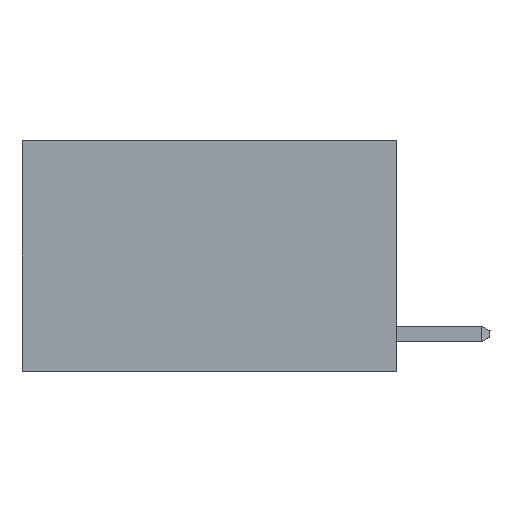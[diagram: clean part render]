
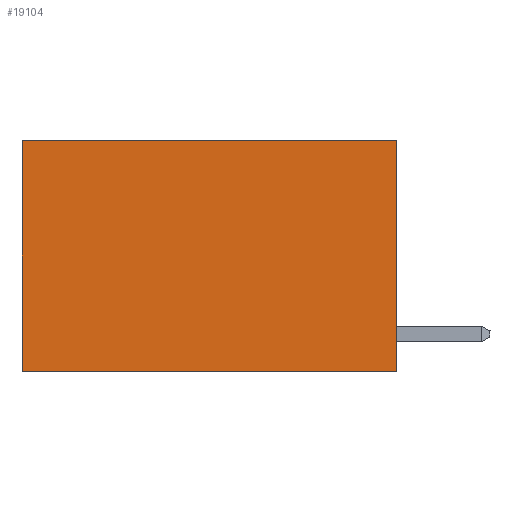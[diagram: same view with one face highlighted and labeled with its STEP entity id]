
A CAD part, left-side view. The second image highlights one B-rep face of the part: STEP entity #19104.
In plain terms, the highlighted planar face has unit normal (-1, 0, 0).
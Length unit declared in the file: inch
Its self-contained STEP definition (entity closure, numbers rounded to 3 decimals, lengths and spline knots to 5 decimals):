
#360 = VERTEX_POINT ( 'NONE', #3849 ) ;
#455 = VERTEX_POINT ( 'NONE', #20634 ) ;
#544 = VECTOR ( 'NONE', #22483, 39.37008 ) ;
#897 = DIRECTION ( 'NONE',  ( 0., 1., 0. ) ) ;
#1497 = ORIENTED_EDGE ( 'NONE', *, *, #5236, .T. ) ;
#1643 = ORIENTED_EDGE ( 'NONE', *, *, #20049, .F. ) ;
#1742 = DIRECTION ( 'NONE',  ( 0., 0., -1. ) ) ;
#2831 = DIRECTION ( 'NONE',  ( 0., 0., -1. ) ) ;
#3849 = CARTESIAN_POINT ( 'NONE',  ( 0.2625, 0., -0.37 ) ) ;
#4881 = ORIENTED_EDGE ( 'NONE', *, *, #5861, .T. ) ;
#5236 = EDGE_CURVE ( 'NONE', #24550, #455, #22586, .T. ) ;
#5306 = FACE_OUTER_BOUND ( 'NONE', #16448, .T. ) ;
#5861 = EDGE_CURVE ( 'NONE', #455, #8704, #11756, .T. ) ;
#6085 = VECTOR ( 'NONE', #17702, 39.37008 ) ;
#8704 = VERTEX_POINT ( 'NONE', #14972 ) ;
#11299 = PLANE ( 'NONE',  #25858 ) ;
#11756 = LINE ( 'NONE', #19719, #6085 ) ;
#13417 = CARTESIAN_POINT ( 'NONE',  ( 0.2625, 0., 0. ) ) ;
#13444 = EDGE_CURVE ( 'NONE', #360, #8704, #17443, .T. ) ;
#13879 = LINE ( 'NONE', #26933, #24299 ) ;
#14972 = CARTESIAN_POINT ( 'NONE',  ( 0.2625, 0.6, -0.37 ) ) ;
#15527 = DIRECTION ( 'NONE',  ( 1., 0., 0. ) ) ;
#16113 = CARTESIAN_POINT ( 'NONE',  ( 0.2625, 0., -0.37 ) ) ;
#16448 = EDGE_LOOP ( 'NONE', ( #4881, #17006, #1643, #1497 ) ) ;
#17006 = ORIENTED_EDGE ( 'NONE', *, *, #13444, .F. ) ;
#17443 = LINE ( 'NONE', #16113, #544 ) ;
#17694 = CARTESIAN_POINT ( 'NONE',  ( 0.2625, 0., 0. ) ) ;
#17702 = DIRECTION ( 'NONE',  ( 0., 0., -1. ) ) ;
#19104 = ADVANCED_FACE ( 'NONE', ( #5306 ), #11299, .F. ) ;
#19719 = CARTESIAN_POINT ( 'NONE',  ( 0.2625, 0.6, 0. ) ) ;
#19832 = CARTESIAN_POINT ( 'NONE',  ( 0.2625, 0., 0. ) ) ;
#20049 = EDGE_CURVE ( 'NONE', #24550, #360, #13879, .T. ) ;
#20634 = CARTESIAN_POINT ( 'NONE',  ( 0.2625, 0.6, 0. ) ) ;
#21947 = VECTOR ( 'NONE', #897, 39.37008 ) ;
#22483 = DIRECTION ( 'NONE',  ( 0., 1., 0. ) ) ;
#22586 = LINE ( 'NONE', #19832, #21947 ) ;
#24299 = VECTOR ( 'NONE', #1742, 39.37008 ) ;
#24550 = VERTEX_POINT ( 'NONE', #17694 ) ;
#25858 = AXIS2_PLACEMENT_3D ( 'NONE', #13417, #15527, #2831 ) ;
#26933 = CARTESIAN_POINT ( 'NONE',  ( 0.2625, 0., 0. ) ) ;
